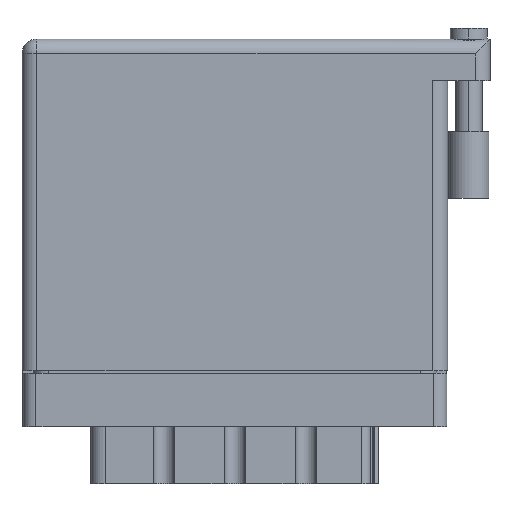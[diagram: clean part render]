
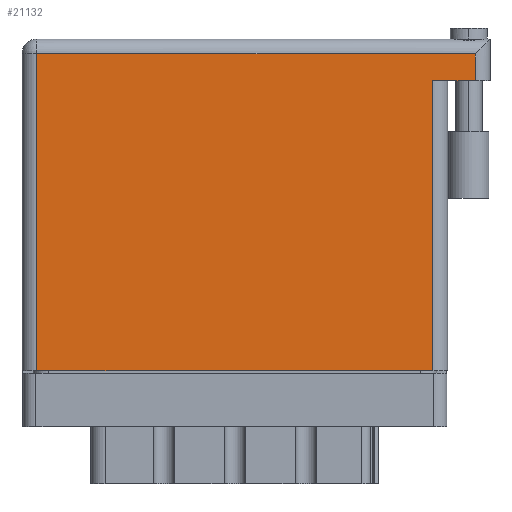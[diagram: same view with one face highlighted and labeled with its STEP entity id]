
A CAD part, front view. The second image highlights one B-rep face of the part: STEP entity #21132.
In plain terms, the highlighted face is planar.
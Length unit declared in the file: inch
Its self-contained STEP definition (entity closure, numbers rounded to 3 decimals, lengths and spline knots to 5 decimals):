
#423 = EDGE_CURVE ( 'NONE', #2754, #26860, #9661, .T. ) ;
#1937 = CARTESIAN_POINT ( 'NONE',  ( 2.138, 1.496, 0. ) ) ;
#2754 = VERTEX_POINT ( 'NONE', #29766 ) ;
#2784 = VECTOR ( 'NONE', #33641, 39.37008 ) ;
#3158 = ORIENTED_EDGE ( 'NONE', *, *, #24599, .T. ) ;
#3269 = LINE ( 'NONE', #17780, #17492 ) ;
#3474 = VECTOR ( 'NONE', #7022, 39.37008 ) ;
#4486 = CARTESIAN_POINT ( 'NONE',  ( 0., 1.566, 0. ) ) ;
#7022 = DIRECTION ( 'NONE',  ( 0., 1., 0. ) ) ;
#7042 = VERTEX_POINT ( 'NONE', #34039 ) ;
#9112 = CARTESIAN_POINT ( 'NONE',  ( 0.07, 0., 0. ) ) ;
#9515 = CARTESIAN_POINT ( 'NONE',  ( 2.138, 1.566, 0. ) ) ;
#9661 = LINE ( 'NONE', #29306, #13654 ) ;
#11026 = VERTEX_POINT ( 'NONE', #15731 ) ;
#13654 = VECTOR ( 'NONE', #15025, 39.37008 ) ;
#14955 = DIRECTION ( 'NONE',  ( 0., 1., 0. ) ) ;
#15025 = DIRECTION ( 'NONE',  ( 0., -1., 0. ) ) ;
#15436 = ORIENTED_EDGE ( 'NONE', *, *, #27658, .T. ) ;
#15731 = CARTESIAN_POINT ( 'NONE',  ( 1.938, 1.369, 0. ) ) ;
#16037 = ORIENTED_EDGE ( 'NONE', *, *, #32540, .T. ) ;
#16261 = AXIS2_PLACEMENT_3D ( 'NONE', #4486, #29819, #24361 ) ;
#16293 = CARTESIAN_POINT ( 'NONE',  ( 0., 1.496, 0. ) ) ;
#17492 = VECTOR ( 'NONE', #14955, 39.37008 ) ;
#17743 = VERTEX_POINT ( 'NONE', #33770 ) ;
#17780 = CARTESIAN_POINT ( 'NONE',  ( 1.938, 1.369, 0. ) ) ;
#18097 = VECTOR ( 'NONE', #36390, 39.37008 ) ;
#18570 = LINE ( 'NONE', #9515, #3474 ) ;
#18880 = DIRECTION ( 'NONE',  ( -1., 0., 0. ) ) ;
#19201 = ORIENTED_EDGE ( 'NONE', *, *, #423, .T. ) ;
#19274 = ORIENTED_EDGE ( 'NONE', *, *, #26769, .T. ) ;
#21132 = ADVANCED_FACE ( 'NONE', ( #33457 ), #21496, .F. ) ;
#21496 = PLANE ( 'NONE',  #16261 ) ;
#21686 = VECTOR ( 'NONE', #18880, 39.37008 ) ;
#22289 = VERTEX_POINT ( 'NONE', #1937 ) ;
#23346 = EDGE_CURVE ( 'NONE', #7042, #11026, #30140, .T. ) ;
#23463 = LINE ( 'NONE', #16293, #21686 ) ;
#24361 = DIRECTION ( 'NONE',  ( -1., 0., 0. ) ) ;
#24599 = EDGE_CURVE ( 'NONE', #22289, #2754, #23463, .T. ) ;
#25008 = LINE ( 'NONE', #27812, #2784 ) ;
#26014 = EDGE_LOOP ( 'NONE', ( #15436, #19274, #35360, #16037, #3158, #19201 ) ) ;
#26769 = EDGE_CURVE ( 'NONE', #17743, #11026, #3269, .T. ) ;
#26860 = VERTEX_POINT ( 'NONE', #9112 ) ;
#27658 = EDGE_CURVE ( 'NONE', #26860, #17743, #25008, .T. ) ;
#27812 = CARTESIAN_POINT ( 'NONE',  ( 0., 0., 0. ) ) ;
#29306 = CARTESIAN_POINT ( 'NONE',  ( 0.07, 0., 0. ) ) ;
#29766 = CARTESIAN_POINT ( 'NONE',  ( 0.07, 1.496, 0. ) ) ;
#29819 = DIRECTION ( 'NONE',  ( 0., 0., -1. ) ) ;
#30140 = LINE ( 'NONE', #33268, #18097 ) ;
#32540 = EDGE_CURVE ( 'NONE', #7042, #22289, #18570, .T. ) ;
#33268 = CARTESIAN_POINT ( 'NONE',  ( 2.208, 1.369, 0. ) ) ;
#33457 = FACE_OUTER_BOUND ( 'NONE', #26014, .T. ) ;
#33641 = DIRECTION ( 'NONE',  ( 1., 0., 0. ) ) ;
#33770 = CARTESIAN_POINT ( 'NONE',  ( 1.938, 0., 0. ) ) ;
#34039 = CARTESIAN_POINT ( 'NONE',  ( 2.138, 1.369, 0. ) ) ;
#35360 = ORIENTED_EDGE ( 'NONE', *, *, #23346, .F. ) ;
#36390 = DIRECTION ( 'NONE',  ( -1., 0., 0. ) ) ;
